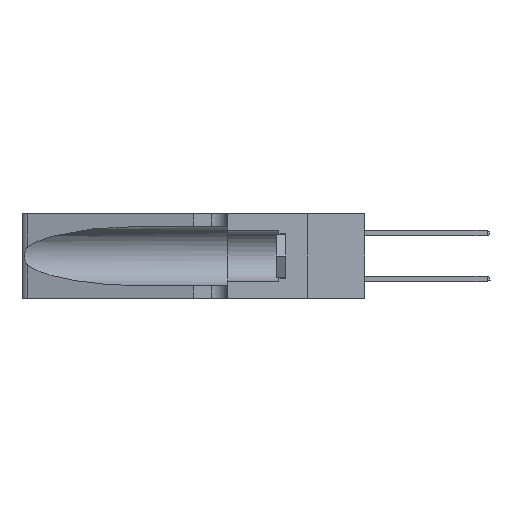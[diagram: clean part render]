
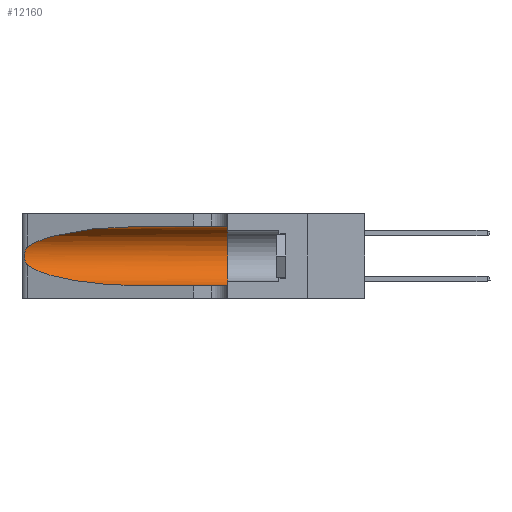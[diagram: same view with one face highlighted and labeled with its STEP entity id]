
A CAD part, left-side view. The second image highlights one B-rep face of the part: STEP entity #12160.
In plain terms, the highlighted cylindrical face has radius 3.308 mm (diameter 6.617 mm), a partial arc.
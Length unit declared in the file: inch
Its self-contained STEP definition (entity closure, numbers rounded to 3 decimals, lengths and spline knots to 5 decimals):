
#100 = AXIS2_PLACEMENT_3D ( 'NONE', #3408, #1393, #24270 ) ;
#171 = EDGE_CURVE ( 'NONE', #13903, #10100, #17305, .T. ) ;
#409 = VERTEX_POINT ( 'NONE', #22824 ) ;
#446 = EDGE_CURVE ( 'NONE', #409, #20687, #26485, .T. ) ;
#683 = VECTOR ( 'NONE', #23892, 39.37008 ) ;
#917 = EDGE_CURVE ( 'NONE', #19054, #20687, #23468, .T. ) ;
#1032 = CARTESIAN_POINT ( 'NONE',  ( 0.25487, 1.22718, 0.14631 ) ) ;
#1088 = CARTESIAN_POINT ( 'NONE',  ( 0.2373, 1.15595, 0.08982 ) ) ;
#1231 = CARTESIAN_POINT ( 'NONE',  ( 0.25639, 1.23184, 0.21858 ) ) ;
#1393 = DIRECTION ( 'NONE',  ( 0., 1., 0. ) ) ;
#2873 = LINE ( 'NONE', #22240, #24684 ) ;
#3408 = CARTESIAN_POINT ( 'NONE',  ( 0.1305, 0.35, 0.185 ) ) ;
#4119 = EDGE_LOOP ( 'NONE', ( #10521, #26135, #19865, #9973, #16147, #26702 ) ) ;
#4446 = DIRECTION ( 'NONE',  ( 0., -1., 0. ) ) ;
#5143 = EDGE_CURVE ( 'NONE', #10100, #19054, #5453, .T. ) ;
#5440 = CARTESIAN_POINT ( 'NONE',  ( 0.26075, 1.23896, 0.19203 ) ) ;
#5453 =( BOUNDED_CURVE ( )  B_SPLINE_CURVE ( 3, ( #15735, #1088, #15824, #20068 ),
 .UNSPECIFIED., .F., .F. ) 
 B_SPLINE_CURVE_WITH_KNOTS ( ( 4, 4 ),
 ( 3.44316, 4.71239 ),
 .UNSPECIFIED. ) 
 CURVE ( )  GEOMETRIC_REPRESENTATION_ITEM ( )  RATIONAL_B_SPLINE_CURVE ( ( 1., 0.87, 0.87, 1. ) ) 
 REPRESENTATION_ITEM ( '' )  );
#5616 = CARTESIAN_POINT ( 'NONE',  ( 0.1305, 0.72297, 0.31525 ) ) ;
#6584 = DIRECTION ( 'NONE',  ( 0., 0., -1. ) ) ;
#7267 = CARTESIAN_POINT ( 'NONE',  ( 0.25555, 1.22994, 0.2215 ) ) ;
#7360 = CARTESIAN_POINT ( 'NONE',  ( 0.25639, 1.23186, 0.15144 ) ) ;
#7550 = CARTESIAN_POINT ( 'NONE',  ( 0.25555, 1.22993, 0.14849 ) ) ;
#8884 = EDGE_CURVE ( 'NONE', #25037, #409, #2873, .T. ) ;
#8939 = CYLINDRICAL_SURFACE ( 'NONE', #10140, 0.13025 ) ;
#9393 = CARTESIAN_POINT ( 'NONE',  ( 0.25487, 1.22718, 0.22369 ) ) ;
#9492 = CARTESIAN_POINT ( 'NONE',  ( 0.25789, 1.23486, 0.15765 ) ) ;
#9712 = CARTESIAN_POINT ( 'NONE',  ( 0.1305, 0.72297, 0.31525 ) ) ;
#9849 = CARTESIAN_POINT ( 'NONE',  ( 0.18966, 0.96281, 0.31525 ) ) ;
#9973 = ORIENTED_EDGE ( 'NONE', *, *, #917, .T. ) ;
#10100 = VERTEX_POINT ( 'NONE', #20006 ) ;
#10140 = AXIS2_PLACEMENT_3D ( 'NONE', #20737, #4446, #6584 ) ;
#10394 = CARTESIAN_POINT ( 'NONE',  ( 0.25487, 1.22718, 0.22369 ) ) ;
#10521 = ORIENTED_EDGE ( 'NONE', *, *, #14035, .T. ) ;
#10982 = CARTESIAN_POINT ( 'NONE',  ( 0.1305, 0.35, 0.05475 ) ) ;
#11916 = CARTESIAN_POINT ( 'NONE',  ( 0.25487, 1.22718, 0.22369 ) ) ;
#12160 = ADVANCED_FACE ( 'NONE', ( #14596 ), #8939, .F. ) ;
#13903 = VERTEX_POINT ( 'NONE', #10394 ) ;
#14035 = EDGE_CURVE ( 'NONE', #25037, #13903, #20698, .T. ) ;
#14202 = CARTESIAN_POINT ( 'NONE',  ( 0.2373, 1.15595, 0.28018 ) ) ;
#14596 = FACE_OUTER_BOUND ( 'NONE', #4119, .T. ) ;
#15590 = CARTESIAN_POINT ( 'NONE',  ( 0.1305, 1.61858, 0.05475 ) ) ;
#15735 = CARTESIAN_POINT ( 'NONE',  ( 0.25487, 1.22718, 0.14631 ) ) ;
#15824 = CARTESIAN_POINT ( 'NONE',  ( 0.18966, 0.96281, 0.05475 ) ) ;
#16147 = ORIENTED_EDGE ( 'NONE', *, *, #446, .F. ) ;
#17305 = B_SPLINE_CURVE_WITH_KNOTS ( 'NONE', 3,
 ( #9393, #7267, #1231, #18096, #26618, #24390, #5440, #20105, #22083, #26418, #9492, #7360, #7550, #1032 ),
 .UNSPECIFIED., .F., .F.,
 ( 4, 2, 2, 2, 2, 2, 4 ),
 ( 0., 0.00027, 0.00053, 0.00107, 0.0016, 0.00187, 0.00214 ),
 .UNSPECIFIED. ) ;
#18096 = CARTESIAN_POINT ( 'NONE',  ( 0.25787, 1.23484, 0.2124 ) ) ;
#19054 = VERTEX_POINT ( 'NONE', #23754 ) ;
#19865 = ORIENTED_EDGE ( 'NONE', *, *, #5143, .T. ) ;
#20006 = CARTESIAN_POINT ( 'NONE',  ( 0.25487, 1.22718, 0.14631 ) ) ;
#20068 = CARTESIAN_POINT ( 'NONE',  ( 0.1305, 0.72297, 0.05475 ) ) ;
#20105 = CARTESIAN_POINT ( 'NONE',  ( 0.26075, 1.23896, 0.178 ) ) ;
#20687 = VERTEX_POINT ( 'NONE', #10982 ) ;
#20698 =( BOUNDED_CURVE ( )  B_SPLINE_CURVE ( 3, ( #5616, #9849, #14202, #11916 ),
 .UNSPECIFIED., .F., .F. ) 
 B_SPLINE_CURVE_WITH_KNOTS ( ( 4, 4 ),
 ( 1.5708, 2.84003 ),
 .UNSPECIFIED. ) 
 CURVE ( )  GEOMETRIC_REPRESENTATION_ITEM ( )  RATIONAL_B_SPLINE_CURVE ( ( 1., 0.87, 0.87, 1. ) ) 
 REPRESENTATION_ITEM ( '' )  );
#20737 = CARTESIAN_POINT ( 'NONE',  ( 0.1305, 1.61858, 0.185 ) ) ;
#22083 = CARTESIAN_POINT ( 'NONE',  ( 0.26017, 1.23833, 0.17102 ) ) ;
#22240 = CARTESIAN_POINT ( 'NONE',  ( 0.1305, 1.61858, 0.31525 ) ) ;
#22824 = CARTESIAN_POINT ( 'NONE',  ( 0.1305, 0.35, 0.31525 ) ) ;
#23468 = LINE ( 'NONE', #15590, #683 ) ;
#23754 = CARTESIAN_POINT ( 'NONE',  ( 0.1305, 0.72297, 0.05475 ) ) ;
#23892 = DIRECTION ( 'NONE',  ( 0., -1., 0. ) ) ;
#24270 = DIRECTION ( 'NONE',  ( 0., 0., 1. ) ) ;
#24390 = CARTESIAN_POINT ( 'NONE',  ( 0.26018, 1.23835, 0.19895 ) ) ;
#24684 = VECTOR ( 'NONE', #26496, 39.37008 ) ;
#25037 = VERTEX_POINT ( 'NONE', #9712 ) ;
#26135 = ORIENTED_EDGE ( 'NONE', *, *, #171, .T. ) ;
#26418 = CARTESIAN_POINT ( 'NONE',  ( 0.25856, 1.23593, 0.16098 ) ) ;
#26485 = CIRCLE ( 'NONE', #100, 0.13025 ) ;
#26496 = DIRECTION ( 'NONE',  ( 0., -1., 0. ) ) ;
#26618 = CARTESIAN_POINT ( 'NONE',  ( 0.25854, 1.2359, 0.20912 ) ) ;
#26702 = ORIENTED_EDGE ( 'NONE', *, *, #8884, .F. ) ;
